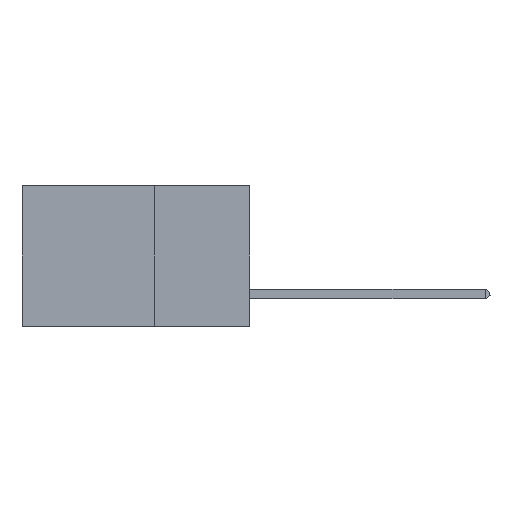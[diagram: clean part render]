
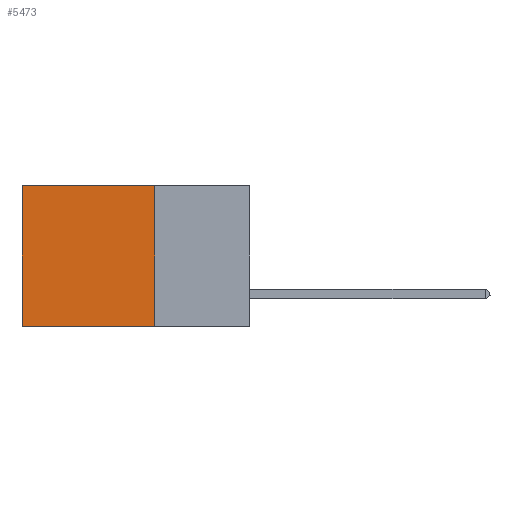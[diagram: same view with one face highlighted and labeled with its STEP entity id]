
A CAD part, left-side view. The second image highlights one B-rep face of the part: STEP entity #5473.
In plain terms, the highlighted planar face has unit normal (-1, 0, 0).
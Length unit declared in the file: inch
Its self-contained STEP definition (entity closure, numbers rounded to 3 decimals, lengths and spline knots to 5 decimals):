
#655 = FACE_OUTER_BOUND ( 'NONE', #9819, .T. ) ;
#1496 = CARTESIAN_POINT ( 'NONE',  ( 0.2875, 0.25, 0. ) ) ;
#1534 = DIRECTION ( 'NONE',  ( 0., 0., -1. ) ) ;
#2005 = ORIENTED_EDGE ( 'NONE', *, *, #15539, .F. ) ;
#4173 = CARTESIAN_POINT ( 'NONE',  ( 0.2875, 0.6, 0. ) ) ;
#4704 = DIRECTION ( 'NONE',  ( 0., 1., 0. ) ) ;
#5092 = PLANE ( 'NONE',  #14040 ) ;
#5473 = ADVANCED_FACE ( 'NONE', ( #655 ), #5092, .F. ) ;
#5907 = DIRECTION ( 'NONE',  ( 0., 0., -1. ) ) ;
#6511 = LINE ( 'NONE', #18411, #19245 ) ;
#8604 = CARTESIAN_POINT ( 'NONE',  ( 0.2875, 0.25, 0. ) ) ;
#9819 = EDGE_LOOP ( 'NONE', ( #12377, #17963, #2005, #14546 ) ) ;
#9901 = CARTESIAN_POINT ( 'NONE',  ( 0.2875, 0.6, -0.37 ) ) ;
#10506 = VERTEX_POINT ( 'NONE', #16865 ) ;
#11357 = VECTOR ( 'NONE', #5907, 39.37008 ) ;
#11360 = DIRECTION ( 'NONE',  ( 0., 1., 0. ) ) ;
#12002 = CARTESIAN_POINT ( 'NONE',  ( 0.2875, 0.25, 0. ) ) ;
#12377 = ORIENTED_EDGE ( 'NONE', *, *, #13662, .T. ) ;
#13005 = VERTEX_POINT ( 'NONE', #9901 ) ;
#13041 = VERTEX_POINT ( 'NONE', #8604 ) ;
#13321 = EDGE_CURVE ( 'NONE', #13858, #13005, #6511, .T. ) ;
#13662 = EDGE_CURVE ( 'NONE', #10506, #13005, #20072, .T. ) ;
#13721 = DIRECTION ( 'NONE',  ( 1., 0., 0. ) ) ;
#13858 = VERTEX_POINT ( 'NONE', #14121 ) ;
#14040 = AXIS2_PLACEMENT_3D ( 'NONE', #1496, #13721, #20483 ) ;
#14121 = CARTESIAN_POINT ( 'NONE',  ( 0.2875, 0.25, -0.37 ) ) ;
#14546 = ORIENTED_EDGE ( 'NONE', *, *, #18873, .T. ) ;
#15029 = LINE ( 'NONE', #12002, #16076 ) ;
#15539 = EDGE_CURVE ( 'NONE', #13041, #13858, #15029, .T. ) ;
#16076 = VECTOR ( 'NONE', #1534, 39.37008 ) ;
#16775 = LINE ( 'NONE', #21908, #21673 ) ;
#16865 = CARTESIAN_POINT ( 'NONE',  ( 0.2875, 0.6, 0. ) ) ;
#17963 = ORIENTED_EDGE ( 'NONE', *, *, #13321, .F. ) ;
#18411 = CARTESIAN_POINT ( 'NONE',  ( 0.2875, 0.25, -0.37 ) ) ;
#18873 = EDGE_CURVE ( 'NONE', #13041, #10506, #16775, .T. ) ;
#19245 = VECTOR ( 'NONE', #11360, 39.37008 ) ;
#20072 = LINE ( 'NONE', #4173, #11357 ) ;
#20483 = DIRECTION ( 'NONE',  ( 0., 0., -1. ) ) ;
#21673 = VECTOR ( 'NONE', #4704, 39.37008 ) ;
#21908 = CARTESIAN_POINT ( 'NONE',  ( 0.2875, 0.25, 0. ) ) ;
